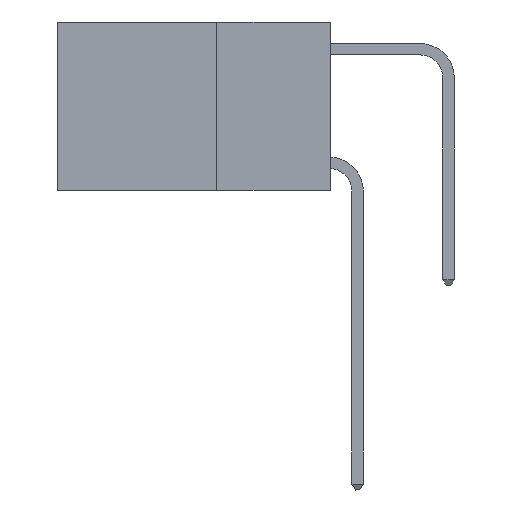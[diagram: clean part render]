
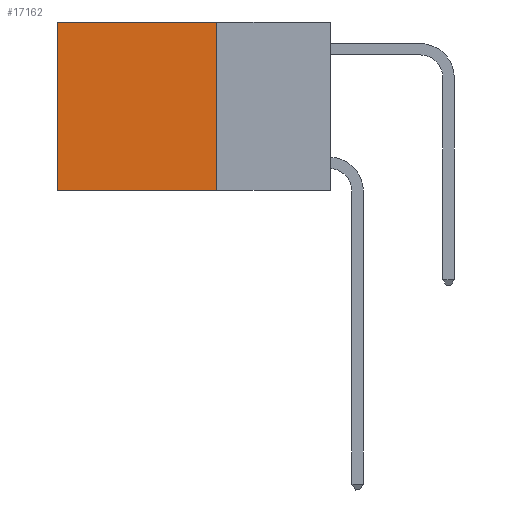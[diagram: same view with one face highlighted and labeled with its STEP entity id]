
A CAD part, left-side view. The second image highlights one B-rep face of the part: STEP entity #17162.
In plain terms, the highlighted planar face has unit normal (-1, 0, 0).
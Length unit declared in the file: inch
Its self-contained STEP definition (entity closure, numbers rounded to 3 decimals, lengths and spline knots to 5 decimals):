
#271 = EDGE_CURVE ( 'NONE', #28687, #29668, #2896, .T. ) ;
#1758 = EDGE_CURVE ( 'NONE', #28687, #26511, #29493, .T. ) ;
#1768 = ORIENTED_EDGE ( 'NONE', *, *, #13984, .F. ) ;
#2896 = LINE ( 'NONE', #16545, #26842 ) ;
#3757 = LINE ( 'NONE', #21496, #11384 ) ;
#4379 = DIRECTION ( 'NONE',  ( 1., 0., 0. ) ) ;
#4738 = EDGE_LOOP ( 'NONE', ( #21798, #1768, #16070, #24401 ) ) ;
#6611 = VECTOR ( 'NONE', #12130, 39.37008 ) ;
#6777 = CARTESIAN_POINT ( 'NONE',  ( 0.2625, 0.6, 0. ) ) ;
#8372 = DIRECTION ( 'NONE',  ( 0., 1., 0. ) ) ;
#9208 = VECTOR ( 'NONE', #8372, 39.37008 ) ;
#9898 = CARTESIAN_POINT ( 'NONE',  ( 0.2625, 0.25, 0. ) ) ;
#11384 = VECTOR ( 'NONE', #18946, 39.37008 ) ;
#11508 = CARTESIAN_POINT ( 'NONE',  ( 0.2625, 0.25, -0.37 ) ) ;
#11832 = VERTEX_POINT ( 'NONE', #30170 ) ;
#12130 = DIRECTION ( 'NONE',  ( 0., 0., -1. ) ) ;
#13439 = LINE ( 'NONE', #29875, #6611 ) ;
#13984 = EDGE_CURVE ( 'NONE', #29668, #11832, #3757, .T. ) ;
#14584 = CARTESIAN_POINT ( 'NONE',  ( 0.2625, 0.25, 0. ) ) ;
#16070 = ORIENTED_EDGE ( 'NONE', *, *, #271, .F. ) ;
#16545 = CARTESIAN_POINT ( 'NONE',  ( 0.2625, 0.25, 0. ) ) ;
#17162 = ADVANCED_FACE ( 'NONE', ( #23975 ), #19686, .F. ) ;
#18946 = DIRECTION ( 'NONE',  ( 0., 1., 0. ) ) ;
#19686 = PLANE ( 'NONE',  #20191 ) ;
#20191 = AXIS2_PLACEMENT_3D ( 'NONE', #14584, #4379, #22227 ) ;
#20984 = EDGE_CURVE ( 'NONE', #26511, #11832, #13439, .T. ) ;
#21037 = CARTESIAN_POINT ( 'NONE',  ( 0.2625, 0.25, 0. ) ) ;
#21496 = CARTESIAN_POINT ( 'NONE',  ( 0.2625, 0.25, -0.37 ) ) ;
#21798 = ORIENTED_EDGE ( 'NONE', *, *, #20984, .T. ) ;
#22227 = DIRECTION ( 'NONE',  ( 0., 0., -1. ) ) ;
#23975 = FACE_OUTER_BOUND ( 'NONE', #4738, .T. ) ;
#24401 = ORIENTED_EDGE ( 'NONE', *, *, #1758, .T. ) ;
#26511 = VERTEX_POINT ( 'NONE', #6777 ) ;
#26842 = VECTOR ( 'NONE', #32084, 39.37008 ) ;
#28687 = VERTEX_POINT ( 'NONE', #9898 ) ;
#29493 = LINE ( 'NONE', #21037, #9208 ) ;
#29668 = VERTEX_POINT ( 'NONE', #11508 ) ;
#29875 = CARTESIAN_POINT ( 'NONE',  ( 0.2625, 0.6, 0. ) ) ;
#30170 = CARTESIAN_POINT ( 'NONE',  ( 0.2625, 0.6, -0.37 ) ) ;
#32084 = DIRECTION ( 'NONE',  ( 0., 0., -1. ) ) ;
